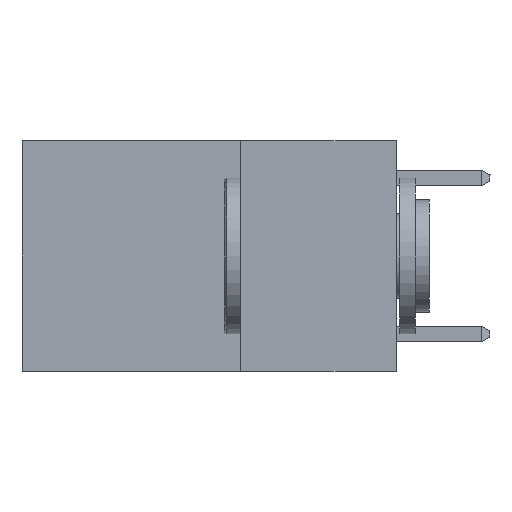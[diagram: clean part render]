
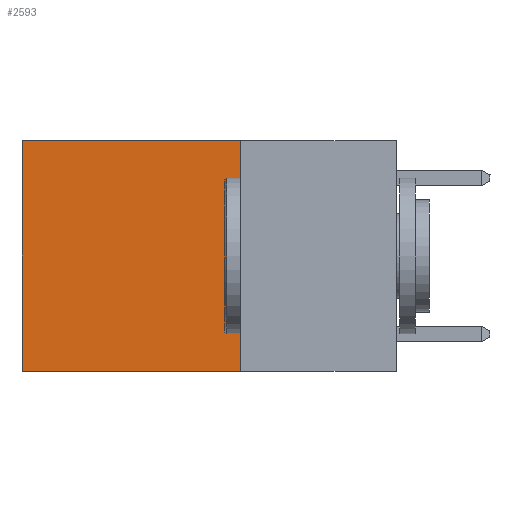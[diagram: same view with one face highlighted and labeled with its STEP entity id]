
A CAD part, left-side view. The second image highlights one B-rep face of the part: STEP entity #2593.
In plain terms, the highlighted planar face has unit normal (-1, 0, 0).
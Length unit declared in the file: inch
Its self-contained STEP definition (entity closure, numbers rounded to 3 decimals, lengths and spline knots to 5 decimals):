
#6 = ORIENTED_EDGE ( 'NONE', *, *, #6338, .F. ) ;
#46 = EDGE_CURVE ( 'NONE', #3916, #6236, #2527, .T. ) ;
#293 = EDGE_LOOP ( 'NONE', ( #6436, #7738, #6, #7143 ) ) ;
#358 = FACE_OUTER_BOUND ( 'NONE', #293, .T. ) ;
#936 = VECTOR ( 'NONE', #9805, 39.37008 ) ;
#1439 = PLANE ( 'NONE',  #8544 ) ;
#1518 = DIRECTION ( 'NONE',  ( 1., 0., 0. ) ) ;
#2214 = EDGE_CURVE ( 'NONE', #9159, #3916, #6021, .T. ) ;
#2527 = LINE ( 'NONE', #3122, #10915 ) ;
#2593 = ADVANCED_FACE ( 'NONE', ( #358 ), #1439, .F. ) ;
#3122 = CARTESIAN_POINT ( 'NONE',  ( 0.2625, 0.6, 0. ) ) ;
#3825 = VECTOR ( 'NONE', #9254, 39.37008 ) ;
#3916 = VERTEX_POINT ( 'NONE', #8729 ) ;
#4184 = VERTEX_POINT ( 'NONE', #8195 ) ;
#4191 = CARTESIAN_POINT ( 'NONE',  ( 0.2625, 0.25, 0. ) ) ;
#6021 = LINE ( 'NONE', #4191, #3825 ) ;
#6236 = VERTEX_POINT ( 'NONE', #10604 ) ;
#6338 = EDGE_CURVE ( 'NONE', #9159, #4184, #9900, .T. ) ;
#6436 = ORIENTED_EDGE ( 'NONE', *, *, #46, .T. ) ;
#6624 = CARTESIAN_POINT ( 'NONE',  ( 0.2625, 0.25, 0. ) ) ;
#6830 = EDGE_CURVE ( 'NONE', #4184, #6236, #7804, .T. ) ;
#7143 = ORIENTED_EDGE ( 'NONE', *, *, #2214, .T. ) ;
#7389 = CARTESIAN_POINT ( 'NONE',  ( 0.2625, 0.25, 0. ) ) ;
#7405 = VECTOR ( 'NONE', #8236, 39.37008 ) ;
#7502 = DIRECTION ( 'NONE',  ( 0., 0., -1. ) ) ;
#7738 = ORIENTED_EDGE ( 'NONE', *, *, #6830, .F. ) ;
#7804 = LINE ( 'NONE', #10623, #936 ) ;
#8195 = CARTESIAN_POINT ( 'NONE',  ( 0.2625, 0.25, -0.37 ) ) ;
#8236 = DIRECTION ( 'NONE',  ( 0., 0., -1. ) ) ;
#8544 = AXIS2_PLACEMENT_3D ( 'NONE', #6624, #1518, #7502 ) ;
#8729 = CARTESIAN_POINT ( 'NONE',  ( 0.2625, 0.6, 0. ) ) ;
#8784 = DIRECTION ( 'NONE',  ( 0., 0., -1. ) ) ;
#9159 = VERTEX_POINT ( 'NONE', #10923 ) ;
#9254 = DIRECTION ( 'NONE',  ( 0., 1., 0. ) ) ;
#9805 = DIRECTION ( 'NONE',  ( 0., 1., 0. ) ) ;
#9900 = LINE ( 'NONE', #7389, #7405 ) ;
#10604 = CARTESIAN_POINT ( 'NONE',  ( 0.2625, 0.6, -0.37 ) ) ;
#10623 = CARTESIAN_POINT ( 'NONE',  ( 0.2625, 0.25, -0.37 ) ) ;
#10915 = VECTOR ( 'NONE', #8784, 39.37008 ) ;
#10923 = CARTESIAN_POINT ( 'NONE',  ( 0.2625, 0.25, 0. ) ) ;
